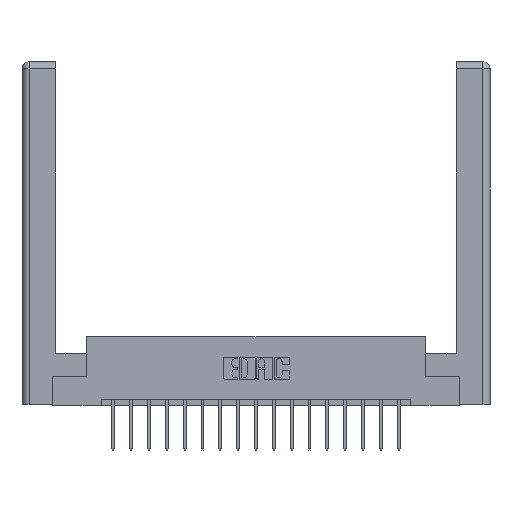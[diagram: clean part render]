
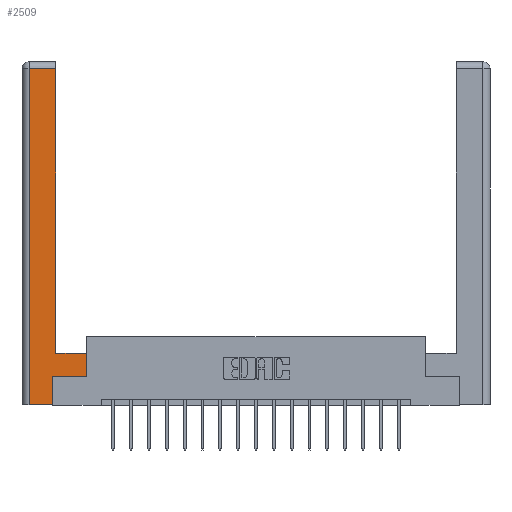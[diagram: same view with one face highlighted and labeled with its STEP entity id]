
A CAD part, top view. The second image highlights one B-rep face of the part: STEP entity #2509.
In plain terms, the highlighted planar face has unit normal (0, 0, 1).
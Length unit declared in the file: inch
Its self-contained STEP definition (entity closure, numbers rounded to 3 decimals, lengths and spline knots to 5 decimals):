
#227 = VECTOR ( 'NONE', #3956, 39.37008 ) ;
#243 = CARTESIAN_POINT ( 'NONE',  ( 0.565, 0.45, 0. ) ) ;
#265 = DIRECTION ( 'NONE',  ( 1., 0., 0. ) ) ;
#280 = CARTESIAN_POINT ( 'NONE',  ( 0.295, 2.94, 0. ) ) ;
#378 = DIRECTION ( 'NONE',  ( 0., 1., 0. ) ) ;
#916 = LINE ( 'NONE', #15385, #3922 ) ;
#1549 = EDGE_CURVE ( 'NONE', #10927, #12532, #5615, .T. ) ;
#1721 = DIRECTION ( 'NONE',  ( 0., 1., 0. ) ) ;
#1815 = VERTEX_POINT ( 'NONE', #2908 ) ;
#1928 = ORIENTED_EDGE ( 'NONE', *, *, #4937, .T. ) ;
#2455 = CARTESIAN_POINT ( 'NONE',  ( 0.0615, 0., 0. ) ) ;
#2509 = ADVANCED_FACE ( 'NONE', ( #9019 ), #10120, .F. ) ;
#2549 = ORIENTED_EDGE ( 'NONE', *, *, #13314, .T. ) ;
#2629 = VERTEX_POINT ( 'NONE', #15063 ) ;
#2652 = DIRECTION ( 'NONE',  ( 1., 0., 0. ) ) ;
#2663 = VECTOR ( 'NONE', #378, 39.37008 ) ;
#2714 = VECTOR ( 'NONE', #4974, 39.37008 ) ;
#2908 = CARTESIAN_POINT ( 'NONE',  ( 0.265, 0., 0. ) ) ;
#3539 = CARTESIAN_POINT ( 'NONE',  ( 0.565, 0.245, 0. ) ) ;
#3546 = EDGE_CURVE ( 'NONE', #16600, #9236, #5761, .T. ) ;
#3775 = DIRECTION ( 'NONE',  ( -1., 0., 0. ) ) ;
#3922 = VECTOR ( 'NONE', #3775, 39.37008 ) ;
#3956 = DIRECTION ( 'NONE',  ( 0., -1., 0. ) ) ;
#4354 = ORIENTED_EDGE ( 'NONE', *, *, #13280, .T. ) ;
#4477 = ORIENTED_EDGE ( 'NONE', *, *, #18434, .T. ) ;
#4843 = CARTESIAN_POINT ( 'NONE',  ( 0.265, 0.245, 0. ) ) ;
#4922 = VECTOR ( 'NONE', #265, 39.37008 ) ;
#4937 = EDGE_CURVE ( 'NONE', #1815, #10927, #18366, .T. ) ;
#4974 = DIRECTION ( 'NONE',  ( -1., 0., 0. ) ) ;
#5615 = LINE ( 'NONE', #16562, #4922 ) ;
#5761 = LINE ( 'NONE', #8717, #2714 ) ;
#6461 = EDGE_CURVE ( 'NONE', #7358, #16600, #17626, .T. ) ;
#7042 = DIRECTION ( 'NONE',  ( 0., 0., -1. ) ) ;
#7193 = ORIENTED_EDGE ( 'NONE', *, *, #9201, .T. ) ;
#7358 = VERTEX_POINT ( 'NONE', #18204 ) ;
#7615 = LINE ( 'NONE', #2455, #227 ) ;
#8118 = AXIS2_PLACEMENT_3D ( 'NONE', #11353, #7042, #11480 ) ;
#8415 = VECTOR ( 'NONE', #15427, 39.37008 ) ;
#8717 = CARTESIAN_POINT ( 'NONE',  ( 0.0615, 2.94, 0. ) ) ;
#9019 = FACE_OUTER_BOUND ( 'NONE', #10949, .T. ) ;
#9201 = EDGE_CURVE ( 'NONE', #12532, #2629, #19050, .T. ) ;
#9236 = VERTEX_POINT ( 'NONE', #13746 ) ;
#10094 = CARTESIAN_POINT ( 'NONE',  ( 0.265, 0., 0. ) ) ;
#10120 = PLANE ( 'NONE',  #8118 ) ;
#10927 = VERTEX_POINT ( 'NONE', #13366 ) ;
#10949 = EDGE_LOOP ( 'NONE', ( #17482, #13143, #2549, #4477, #1928, #16398, #7193, #4354 ) ) ;
#11231 = VECTOR ( 'NONE', #1721, 39.37008 ) ;
#11353 = CARTESIAN_POINT ( 'NONE',  ( 0., 0., 0. ) ) ;
#11480 = DIRECTION ( 'NONE',  ( -1., 0., 0. ) ) ;
#12030 = CARTESIAN_POINT ( 'NONE',  ( 0.0615, 0., 0. ) ) ;
#12269 = CARTESIAN_POINT ( 'NONE',  ( 0.295, 3., 0. ) ) ;
#12532 = VERTEX_POINT ( 'NONE', #3539 ) ;
#13143 = ORIENTED_EDGE ( 'NONE', *, *, #3546, .T. ) ;
#13280 = EDGE_CURVE ( 'NONE', #2629, #7358, #916, .T. ) ;
#13314 = EDGE_CURVE ( 'NONE', #9236, #14688, #7615, .T. ) ;
#13366 = CARTESIAN_POINT ( 'NONE',  ( 0.265, 0.245, 0. ) ) ;
#13746 = CARTESIAN_POINT ( 'NONE',  ( 0.0615, 2.94, 0. ) ) ;
#14688 = VERTEX_POINT ( 'NONE', #12030 ) ;
#15063 = CARTESIAN_POINT ( 'NONE',  ( 0.565, 0.45, 0. ) ) ;
#15385 = CARTESIAN_POINT ( 'NONE',  ( 0.295, 0.45, 0. ) ) ;
#15427 = DIRECTION ( 'NONE',  ( 0., 1., 0. ) ) ;
#16398 = ORIENTED_EDGE ( 'NONE', *, *, #1549, .T. ) ;
#16562 = CARTESIAN_POINT ( 'NONE',  ( 0.565, 0.245, 0. ) ) ;
#16600 = VERTEX_POINT ( 'NONE', #280 ) ;
#16628 = LINE ( 'NONE', #10094, #17325 ) ;
#17325 = VECTOR ( 'NONE', #2652, 39.37008 ) ;
#17482 = ORIENTED_EDGE ( 'NONE', *, *, #6461, .T. ) ;
#17626 = LINE ( 'NONE', #12269, #8415 ) ;
#18204 = CARTESIAN_POINT ( 'NONE',  ( 0.295, 0.45, 0. ) ) ;
#18366 = LINE ( 'NONE', #4843, #2663 ) ;
#18434 = EDGE_CURVE ( 'NONE', #14688, #1815, #16628, .T. ) ;
#19050 = LINE ( 'NONE', #243, #11231 ) ;
